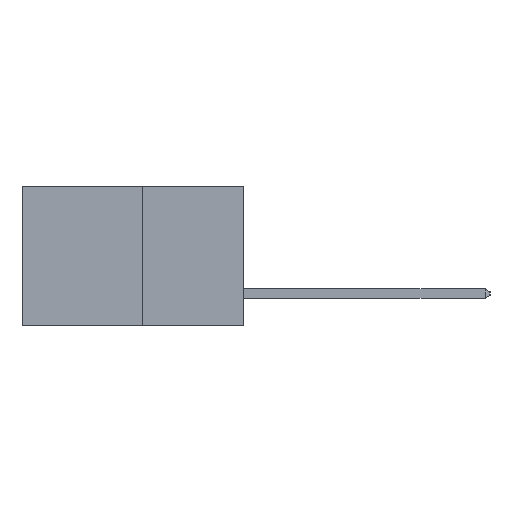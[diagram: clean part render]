
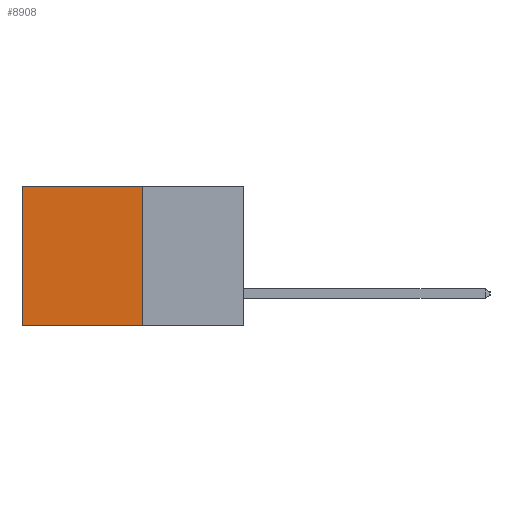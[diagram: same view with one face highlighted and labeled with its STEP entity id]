
A CAD part, left-side view. The second image highlights one B-rep face of the part: STEP entity #8908.
In plain terms, the highlighted planar face has unit normal (-1, 0, 0).
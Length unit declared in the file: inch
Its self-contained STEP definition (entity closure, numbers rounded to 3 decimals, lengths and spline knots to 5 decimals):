
#216 = CARTESIAN_POINT ( 'NONE',  ( 0.277, 0.27, 0. ) ) ;
#322 = EDGE_CURVE ( 'NONE', #7555, #1411, #583, .T. ) ;
#583 = LINE ( 'NONE', #4327, #8051 ) ;
#995 = VERTEX_POINT ( 'NONE', #2694 ) ;
#1034 = LINE ( 'NONE', #7449, #8238 ) ;
#1294 = DIRECTION ( 'NONE',  ( 1., 0., 0. ) ) ;
#1411 = VERTEX_POINT ( 'NONE', #2068 ) ;
#1476 = AXIS2_PLACEMENT_3D ( 'NONE', #9051, #1294, #6427 ) ;
#2068 = CARTESIAN_POINT ( 'NONE',  ( 0.277, 0.27, -0.37 ) ) ;
#2365 = CARTESIAN_POINT ( 'NONE',  ( 0.277, 0.27, 0. ) ) ;
#2483 = CARTESIAN_POINT ( 'NONE',  ( 0.277, 0.59, -0.37 ) ) ;
#2694 = CARTESIAN_POINT ( 'NONE',  ( 0.277, 0.59, 0. ) ) ;
#3125 = DIRECTION ( 'NONE',  ( 0., 0., -1. ) ) ;
#3319 = LINE ( 'NONE', #216, #9076 ) ;
#4197 = PLANE ( 'NONE',  #1476 ) ;
#4327 = CARTESIAN_POINT ( 'NONE',  ( 0.277, 0.27, -0.37 ) ) ;
#4366 = ORIENTED_EDGE ( 'NONE', *, *, #8697, .T. ) ;
#4421 = VERTEX_POINT ( 'NONE', #5724 ) ;
#4431 = ORIENTED_EDGE ( 'NONE', *, *, #6376, .F. ) ;
#4487 = ORIENTED_EDGE ( 'NONE', *, *, #322, .F. ) ;
#4494 = ORIENTED_EDGE ( 'NONE', *, *, #8296, .T. ) ;
#4740 = DIRECTION ( 'NONE',  ( 0., 0., -1. ) ) ;
#5724 = CARTESIAN_POINT ( 'NONE',  ( 0.277, 0.59, -0.37 ) ) ;
#5959 = FACE_OUTER_BOUND ( 'NONE', #6023, .T. ) ;
#6023 = EDGE_LOOP ( 'NONE', ( #4366, #4431, #4487, #4494 ) ) ;
#6089 = VECTOR ( 'NONE', #4740, 39.37008 ) ;
#6376 = EDGE_CURVE ( 'NONE', #1411, #4421, #1034, .T. ) ;
#6427 = DIRECTION ( 'NONE',  ( 0., 0., -1. ) ) ;
#7449 = CARTESIAN_POINT ( 'NONE',  ( 0.277, 0.27, -0.37 ) ) ;
#7467 = DIRECTION ( 'NONE',  ( 0., 1., 0. ) ) ;
#7555 = VERTEX_POINT ( 'NONE', #2365 ) ;
#7847 = DIRECTION ( 'NONE',  ( 0., 1., 0. ) ) ;
#7929 = LINE ( 'NONE', #2483, #6089 ) ;
#8051 = VECTOR ( 'NONE', #3125, 39.37008 ) ;
#8238 = VECTOR ( 'NONE', #7467, 39.37008 ) ;
#8296 = EDGE_CURVE ( 'NONE', #7555, #995, #3319, .T. ) ;
#8697 = EDGE_CURVE ( 'NONE', #995, #4421, #7929, .T. ) ;
#8908 = ADVANCED_FACE ( 'NONE', ( #5959 ), #4197, .F. ) ;
#9051 = CARTESIAN_POINT ( 'NONE',  ( 0.277, 0.27, -0.37 ) ) ;
#9076 = VECTOR ( 'NONE', #7847, 39.37008 ) ;
